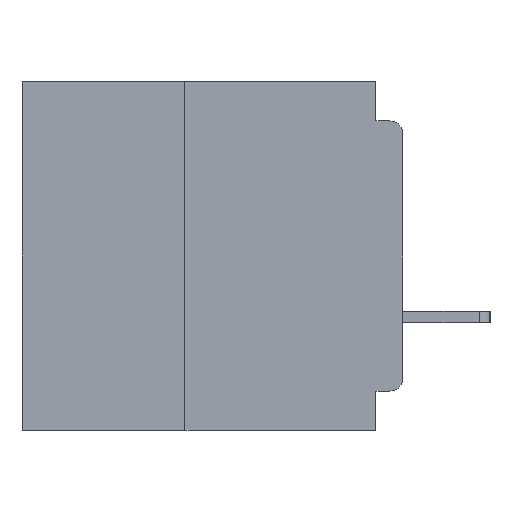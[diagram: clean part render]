
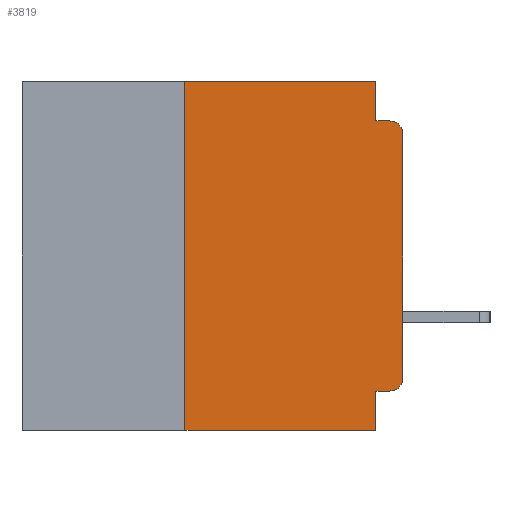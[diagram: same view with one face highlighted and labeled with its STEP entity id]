
A CAD part, left-side view. The second image highlights one B-rep face of the part: STEP entity #3819.
In plain terms, the highlighted planar face has unit normal (-1, 0, 0).
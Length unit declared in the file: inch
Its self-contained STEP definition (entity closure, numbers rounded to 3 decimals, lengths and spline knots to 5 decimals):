
#526 = EDGE_CURVE ( 'NONE', #42388, #58025, #46752, .T. ) ;
#930 = CARTESIAN_POINT ( 'NONE',  ( 0., 0.25, -0.4 ) ) ;
#1305 = VERTEX_POINT ( 'NONE', #58829 ) ;
#1466 = VERTEX_POINT ( 'NONE', #53230 ) ;
#2880 = LINE ( 'NONE', #54358, #14998 ) ;
#3129 = CARTESIAN_POINT ( 'NONE',  ( 0., 0.031, -0.4 ) ) ;
#3819 = ADVANCED_FACE ( 'NONE', ( #31598 ), #14326, .F. ) ;
#3891 = LINE ( 'NONE', #46348, #26634 ) ;
#4058 = VERTEX_POINT ( 'NONE', #930 ) ;
#4430 = CARTESIAN_POINT ( 'NONE',  ( 0., 0.031, -0.4 ) ) ;
#4669 = ORIENTED_EDGE ( 'NONE', *, *, #40798, .F. ) ;
#5612 = VERTEX_POINT ( 'NONE', #17697 ) ;
#6988 = EDGE_CURVE ( 'NONE', #1305, #12485, #47199, .T. ) ;
#7366 = VERTEX_POINT ( 'NONE', #25450 ) ;
#7415 = CARTESIAN_POINT ( 'NONE',  ( 0., 0.031, 0. ) ) ;
#8719 = DIRECTION ( 'NONE',  ( 0., -1., 0. ) ) ;
#8754 = ORIENTED_EDGE ( 'NONE', *, *, #25443, .F. ) ;
#9210 = CIRCLE ( 'NONE', #50292, 0.015 ) ;
#9431 = DIRECTION ( 'NONE',  ( 0., 0., 1. ) ) ;
#11058 = VECTOR ( 'NONE', #49651, 39.37008 ) ;
#12261 = DIRECTION ( 'NONE',  ( -1., 0., 0. ) ) ;
#12485 = VERTEX_POINT ( 'NONE', #3129 ) ;
#12538 = DIRECTION ( 'NONE',  ( 0., 0., -1. ) ) ;
#12604 = DIRECTION ( 'NONE',  ( 1., 0., 0. ) ) ;
#13094 = CARTESIAN_POINT ( 'NONE',  ( 0., 0.437, 0. ) ) ;
#13839 = DIRECTION ( 'NONE',  ( 0., -1., 0. ) ) ;
#14326 = PLANE ( 'NONE',  #36655 ) ;
#14998 = VECTOR ( 'NONE', #58869, 39.37008 ) ;
#16599 = EDGE_CURVE ( 'NONE', #5612, #1466, #45815, .T. ) ;
#17697 = CARTESIAN_POINT ( 'NONE',  ( 0., 0., -0.34 ) ) ;
#18087 = LINE ( 'NONE', #20546, #40762 ) ;
#19238 = DIRECTION ( 'NONE',  ( 0., 0., 1. ) ) ;
#20546 = CARTESIAN_POINT ( 'NONE',  ( 0., 0., -0.355 ) ) ;
#22446 = CARTESIAN_POINT ( 'NONE',  ( 0., 0.25, 0. ) ) ;
#22910 = EDGE_CURVE ( 'NONE', #7366, #5612, #47235, .T. ) ;
#23881 = DIRECTION ( 'NONE',  ( 0., -1., 0. ) ) ;
#24342 = DIRECTION ( 'NONE',  ( -1., 0., 0. ) ) ;
#24938 = EDGE_CURVE ( 'NONE', #25423, #35151, #40579, .T. ) ;
#25423 = VERTEX_POINT ( 'NONE', #22446 ) ;
#25443 = EDGE_CURVE ( 'NONE', #35151, #42388, #2880, .T. ) ;
#25450 = CARTESIAN_POINT ( 'NONE',  ( 0., 0.015, -0.355 ) ) ;
#26386 = EDGE_CURVE ( 'NONE', #1466, #58025, #9210, .T. ) ;
#26634 = VECTOR ( 'NONE', #19238, 39.37008 ) ;
#28125 = EDGE_LOOP ( 'NONE', ( #36326, #51758, #44500, #8754, #46511, #4669, #36014, #34052, #43177, #48844 ) ) ;
#28563 = VECTOR ( 'NONE', #23881, 39.37008 ) ;
#30119 = LINE ( 'NONE', #45546, #52756 ) ;
#31052 = CARTESIAN_POINT ( 'NONE',  ( 0., 0.015, -0.045 ) ) ;
#31598 = FACE_OUTER_BOUND ( 'NONE', #28125, .T. ) ;
#32505 = CARTESIAN_POINT ( 'NONE',  ( 0., 0., -0.045 ) ) ;
#34052 = ORIENTED_EDGE ( 'NONE', *, *, #6988, .F. ) ;
#34202 = EDGE_CURVE ( 'NONE', #4058, #12485, #30119, .T. ) ;
#34779 = VECTOR ( 'NONE', #8719, 39.37008 ) ;
#35151 = VERTEX_POINT ( 'NONE', #7415 ) ;
#35716 = AXIS2_PLACEMENT_3D ( 'NONE', #51518, #24342, #56056 ) ;
#36014 = ORIENTED_EDGE ( 'NONE', *, *, #34202, .T. ) ;
#36326 = ORIENTED_EDGE ( 'NONE', *, *, #16599, .T. ) ;
#36594 = CARTESIAN_POINT ( 'NONE',  ( 0., 0., 0. ) ) ;
#36629 = VECTOR ( 'NONE', #9431, 39.37008 ) ;
#36655 = AXIS2_PLACEMENT_3D ( 'NONE', #13094, #12604, #12538 ) ;
#39424 = CARTESIAN_POINT ( 'NONE',  ( 0., 0.015, -0.06 ) ) ;
#39751 = EDGE_CURVE ( 'NONE', #7366, #1305, #18087, .T. ) ;
#40579 = LINE ( 'NONE', #51057, #28563 ) ;
#40762 = VECTOR ( 'NONE', #52251, 39.37008 ) ;
#40798 = EDGE_CURVE ( 'NONE', #4058, #25423, #3891, .T. ) ;
#42388 = VERTEX_POINT ( 'NONE', #55633 ) ;
#43177 = ORIENTED_EDGE ( 'NONE', *, *, #39751, .F. ) ;
#43946 = DIRECTION ( 'NONE',  ( 0., 0., -1. ) ) ;
#44500 = ORIENTED_EDGE ( 'NONE', *, *, #526, .F. ) ;
#45546 = CARTESIAN_POINT ( 'NONE',  ( 0., 0.437, -0.4 ) ) ;
#45815 = LINE ( 'NONE', #36594, #36629 ) ;
#46348 = CARTESIAN_POINT ( 'NONE',  ( 0., 0.25, -0.4 ) ) ;
#46511 = ORIENTED_EDGE ( 'NONE', *, *, #24938, .F. ) ;
#46752 = LINE ( 'NONE', #32505, #34779 ) ;
#47199 = LINE ( 'NONE', #4430, #11058 ) ;
#47235 = CIRCLE ( 'NONE', #35716, 0.015 ) ;
#48844 = ORIENTED_EDGE ( 'NONE', *, *, #22910, .T. ) ;
#49651 = DIRECTION ( 'NONE',  ( 0., 0., -1. ) ) ;
#50292 = AXIS2_PLACEMENT_3D ( 'NONE', #39424, #12261, #43946 ) ;
#51057 = CARTESIAN_POINT ( 'NONE',  ( 0., 0.437, 0. ) ) ;
#51518 = CARTESIAN_POINT ( 'NONE',  ( 0., 0.015, -0.34 ) ) ;
#51758 = ORIENTED_EDGE ( 'NONE', *, *, #26386, .T. ) ;
#52251 = DIRECTION ( 'NONE',  ( 0., 1., 0. ) ) ;
#52756 = VECTOR ( 'NONE', #13839, 39.37008 ) ;
#53230 = CARTESIAN_POINT ( 'NONE',  ( 0., 0., -0.06 ) ) ;
#54358 = CARTESIAN_POINT ( 'NONE',  ( 0., 0.031, 0. ) ) ;
#55633 = CARTESIAN_POINT ( 'NONE',  ( 0., 0.031, -0.045 ) ) ;
#56056 = DIRECTION ( 'NONE',  ( 0., 0., -1. ) ) ;
#58025 = VERTEX_POINT ( 'NONE', #31052 ) ;
#58829 = CARTESIAN_POINT ( 'NONE',  ( 0., 0.031, -0.355 ) ) ;
#58869 = DIRECTION ( 'NONE',  ( 0., 0., -1. ) ) ;
